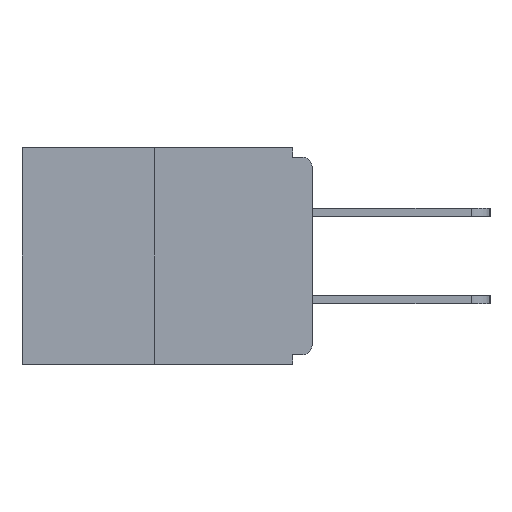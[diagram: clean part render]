
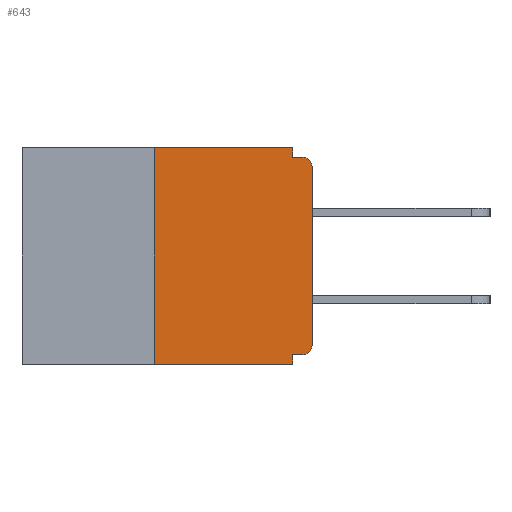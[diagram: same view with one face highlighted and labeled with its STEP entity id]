
A CAD part, left-side view. The second image highlights one B-rep face of the part: STEP entity #643.
In plain terms, the highlighted planar face has unit normal (-1, 0, 0).
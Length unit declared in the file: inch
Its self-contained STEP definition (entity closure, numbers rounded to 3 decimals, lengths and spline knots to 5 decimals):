
#196 = EDGE_CURVE ( 'NONE', #5898, #9736, #7736, .T. ) ;
#219 = LINE ( 'NONE', #10691, #4981 ) ;
#305 = VERTEX_POINT ( 'NONE', #11696 ) ;
#443 = VECTOR ( 'NONE', #4846, 39.37008 ) ;
#510 = CARTESIAN_POINT ( 'NONE',  ( 0., 0.031, -0.015 ) ) ;
#577 = LINE ( 'NONE', #5855, #2803 ) ;
#643 = ADVANCED_FACE ( 'NONE', ( #2475 ), #5801, .F. ) ;
#713 = CARTESIAN_POINT ( 'NONE',  ( 0., 0.031, 0. ) ) ;
#770 = EDGE_CURVE ( 'NONE', #9736, #3960, #577, .T. ) ;
#863 = CARTESIAN_POINT ( 'NONE',  ( 0., 0.25, 0. ) ) ;
#1071 = DIRECTION ( 'NONE',  ( 0., 0., -1. ) ) ;
#1128 = ORIENTED_EDGE ( 'NONE', *, *, #2079, .T. ) ;
#1327 = CARTESIAN_POINT ( 'NONE',  ( 0., 0.015, -0.015 ) ) ;
#1387 = VERTEX_POINT ( 'NONE', #5173 ) ;
#1486 = AXIS2_PLACEMENT_3D ( 'NONE', #10725, #7861, #1789 ) ;
#1494 = CARTESIAN_POINT ( 'NONE',  ( 0., 0.25, -0.343 ) ) ;
#1520 = VERTEX_POINT ( 'NONE', #6454 ) ;
#1565 = ORIENTED_EDGE ( 'NONE', *, *, #9124, .F. ) ;
#1789 = DIRECTION ( 'NONE',  ( 0., 0., -1. ) ) ;
#2076 = EDGE_LOOP ( 'NONE', ( #12361, #12291, #1128, #1565, #5864, #5525, #10762, #4943, #2994, #3072 ) ) ;
#2079 = EDGE_CURVE ( 'NONE', #5898, #1520, #219, .T. ) ;
#2164 = DIRECTION ( 'NONE',  ( 0., 0., -1. ) ) ;
#2179 = LINE ( 'NONE', #2940, #443 ) ;
#2351 = AXIS2_PLACEMENT_3D ( 'NONE', #9205, #5503, #1071 ) ;
#2355 = CARTESIAN_POINT ( 'NONE',  ( 0., 0.015, -0.328 ) ) ;
#2475 = FACE_OUTER_BOUND ( 'NONE', #2076, .T. ) ;
#2589 = EDGE_CURVE ( 'NONE', #10644, #7398, #7049, .T. ) ;
#2709 = VECTOR ( 'NONE', #2164, 39.37008 ) ;
#2803 = VECTOR ( 'NONE', #2841, 39.37008 ) ;
#2841 = DIRECTION ( 'NONE',  ( 0., -1., 0. ) ) ;
#2940 = CARTESIAN_POINT ( 'NONE',  ( 0., 0., -0.015 ) ) ;
#2994 = ORIENTED_EDGE ( 'NONE', *, *, #6281, .F. ) ;
#3072 = ORIENTED_EDGE ( 'NONE', *, *, #5248, .F. ) ;
#3108 = DIRECTION ( 'NONE',  ( 0., 0., -1. ) ) ;
#3960 = VERTEX_POINT ( 'NONE', #713 ) ;
#4038 = AXIS2_PLACEMENT_3D ( 'NONE', #6178, #7168, #3108 ) ;
#4846 = DIRECTION ( 'NONE',  ( 0., -1., 0. ) ) ;
#4943 = ORIENTED_EDGE ( 'NONE', *, *, #9436, .T. ) ;
#4981 = VECTOR ( 'NONE', #6769, 39.37008 ) ;
#5018 = CIRCLE ( 'NONE', #4038, 0.015 ) ;
#5173 = CARTESIAN_POINT ( 'NONE',  ( 0., 0., -0.03 ) ) ;
#5248 = EDGE_CURVE ( 'NONE', #3960, #11836, #5529, .T. ) ;
#5294 = EDGE_CURVE ( 'NONE', #305, #1387, #9184, .T. ) ;
#5503 = DIRECTION ( 'NONE',  ( -1., 0., 0. ) ) ;
#5525 = ORIENTED_EDGE ( 'NONE', *, *, #11644, .T. ) ;
#5529 = LINE ( 'NONE', #10189, #7939 ) ;
#5801 = PLANE ( 'NONE',  #1486 ) ;
#5855 = CARTESIAN_POINT ( 'NONE',  ( 0., 0.46, 0. ) ) ;
#5864 = ORIENTED_EDGE ( 'NONE', *, *, #2589, .F. ) ;
#5898 = VERTEX_POINT ( 'NONE', #1494 ) ;
#6178 = CARTESIAN_POINT ( 'NONE',  ( 0., 0.015, -0.313 ) ) ;
#6281 = EDGE_CURVE ( 'NONE', #11836, #11712, #2179, .T. ) ;
#6454 = CARTESIAN_POINT ( 'NONE',  ( 0., 0.031, -0.343 ) ) ;
#6769 = DIRECTION ( 'NONE',  ( 0., -1., 0. ) ) ;
#6848 = LINE ( 'NONE', #8052, #2709 ) ;
#7049 = LINE ( 'NONE', #9599, #8789 ) ;
#7168 = DIRECTION ( 'NONE',  ( -1., 0., 0. ) ) ;
#7398 = VERTEX_POINT ( 'NONE', #12959 ) ;
#7535 = DIRECTION ( 'NONE',  ( 0., 0., 1. ) ) ;
#7620 = CIRCLE ( 'NONE', #2351, 0.015 ) ;
#7736 = LINE ( 'NONE', #863, #12766 ) ;
#7861 = DIRECTION ( 'NONE',  ( 1., 0., 0. ) ) ;
#7939 = VECTOR ( 'NONE', #10147, 39.37008 ) ;
#8021 = CARTESIAN_POINT ( 'NONE',  ( 0., 0., 0. ) ) ;
#8052 = CARTESIAN_POINT ( 'NONE',  ( 0., 0.031, -0.343 ) ) ;
#8385 = VECTOR ( 'NONE', #10085, 39.37008 ) ;
#8789 = VECTOR ( 'NONE', #10783, 39.37008 ) ;
#9124 = EDGE_CURVE ( 'NONE', #7398, #1520, #6848, .T. ) ;
#9184 = LINE ( 'NONE', #8021, #8385 ) ;
#9205 = CARTESIAN_POINT ( 'NONE',  ( 0., 0.015, -0.03 ) ) ;
#9436 = EDGE_CURVE ( 'NONE', #1387, #11712, #7620, .T. ) ;
#9599 = CARTESIAN_POINT ( 'NONE',  ( 0., 0., -0.328 ) ) ;
#9736 = VERTEX_POINT ( 'NONE', #11048 ) ;
#10085 = DIRECTION ( 'NONE',  ( 0., 0., 1. ) ) ;
#10147 = DIRECTION ( 'NONE',  ( 0., 0., -1. ) ) ;
#10189 = CARTESIAN_POINT ( 'NONE',  ( 0., 0.031, 0. ) ) ;
#10644 = VERTEX_POINT ( 'NONE', #2355 ) ;
#10691 = CARTESIAN_POINT ( 'NONE',  ( 0., 0.46, -0.343 ) ) ;
#10725 = CARTESIAN_POINT ( 'NONE',  ( 0., 0.46, 0. ) ) ;
#10762 = ORIENTED_EDGE ( 'NONE', *, *, #5294, .T. ) ;
#10783 = DIRECTION ( 'NONE',  ( 0., 1., 0. ) ) ;
#11048 = CARTESIAN_POINT ( 'NONE',  ( 0., 0.25, 0. ) ) ;
#11644 = EDGE_CURVE ( 'NONE', #10644, #305, #5018, .T. ) ;
#11696 = CARTESIAN_POINT ( 'NONE',  ( 0., 0., -0.313 ) ) ;
#11712 = VERTEX_POINT ( 'NONE', #1327 ) ;
#11836 = VERTEX_POINT ( 'NONE', #510 ) ;
#12291 = ORIENTED_EDGE ( 'NONE', *, *, #196, .F. ) ;
#12361 = ORIENTED_EDGE ( 'NONE', *, *, #770, .F. ) ;
#12766 = VECTOR ( 'NONE', #7535, 39.37008 ) ;
#12959 = CARTESIAN_POINT ( 'NONE',  ( 0., 0.031, -0.328 ) ) ;
